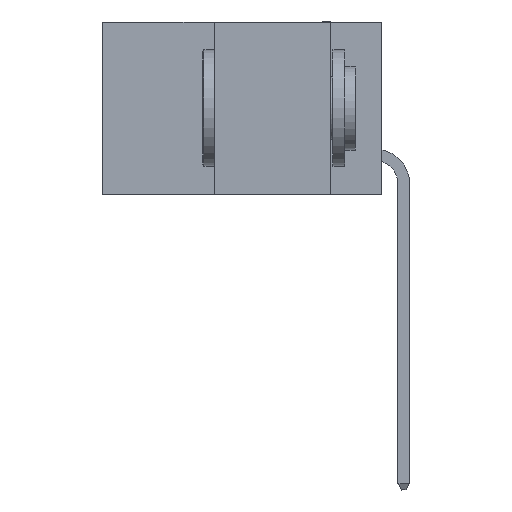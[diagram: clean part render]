
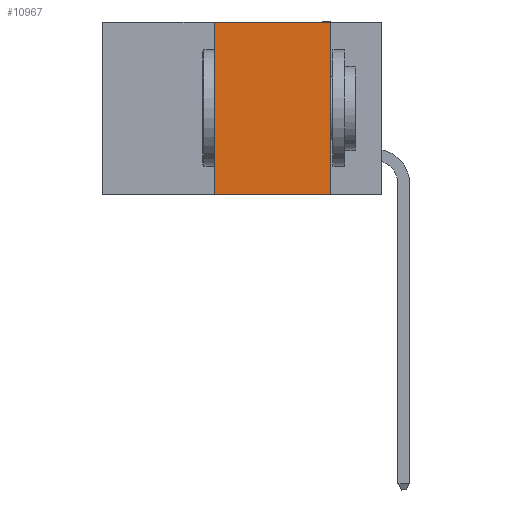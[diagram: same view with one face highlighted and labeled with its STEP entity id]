
A CAD part, left-side view. The second image highlights one B-rep face of the part: STEP entity #10967.
In plain terms, the highlighted planar face has unit normal (-1, 0, 0).
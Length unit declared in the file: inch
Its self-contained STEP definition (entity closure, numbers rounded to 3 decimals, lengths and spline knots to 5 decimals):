
#466 = VECTOR ( 'NONE', #10156, 39.37008 ) ;
#574 = DIRECTION ( 'NONE',  ( 0., 0., 1. ) ) ;
#3462 = CARTESIAN_POINT ( 'NONE',  ( 0., 0.11, -0.37 ) ) ;
#4355 = EDGE_CURVE ( 'NONE', #12598, #27867, #10613, .T. ) ;
#9009 = ORIENTED_EDGE ( 'NONE', *, *, #15326, .F. ) ;
#9457 = CARTESIAN_POINT ( 'NONE',  ( 0., 0.11, 0. ) ) ;
#9523 = DIRECTION ( 'NONE',  ( 1., 0., 0. ) ) ;
#10093 = EDGE_CURVE ( 'NONE', #23717, #25886, #20164, .T. ) ;
#10156 = DIRECTION ( 'NONE',  ( 0., -1., 0. ) ) ;
#10324 = VECTOR ( 'NONE', #28704, 39.37008 ) ;
#10613 = LINE ( 'NONE', #15446, #466 ) ;
#10967 = ADVANCED_FACE ( 'NONE', ( #32724 ), #17359, .F. ) ;
#12266 = VECTOR ( 'NONE', #574, 39.37008 ) ;
#12590 = CARTESIAN_POINT ( 'NONE',  ( 0., 0.6, 0. ) ) ;
#12598 = VERTEX_POINT ( 'NONE', #34914 ) ;
#13986 = CARTESIAN_POINT ( 'NONE',  ( 0., 0.36, 0. ) ) ;
#14071 = CARTESIAN_POINT ( 'NONE',  ( 0., 0.11, 0. ) ) ;
#15326 = EDGE_CURVE ( 'NONE', #25886, #27867, #15802, .T. ) ;
#15446 = CARTESIAN_POINT ( 'NONE',  ( 0., 0.6, -0.37 ) ) ;
#15802 = LINE ( 'NONE', #9457, #10324 ) ;
#17359 = PLANE ( 'NONE',  #34190 ) ;
#19769 = CARTESIAN_POINT ( 'NONE',  ( 0., 0.36, 0. ) ) ;
#20144 = ORIENTED_EDGE ( 'NONE', *, *, #10093, .F. ) ;
#20164 = LINE ( 'NONE', #12590, #30265 ) ;
#23717 = VERTEX_POINT ( 'NONE', #13986 ) ;
#25610 = CARTESIAN_POINT ( 'NONE',  ( 0., 0.6, 0. ) ) ;
#25886 = VERTEX_POINT ( 'NONE', #14071 ) ;
#27046 = EDGE_LOOP ( 'NONE', ( #9009, #20144, #30380, #33128 ) ) ;
#27867 = VERTEX_POINT ( 'NONE', #3462 ) ;
#28590 = EDGE_CURVE ( 'NONE', #12598, #23717, #32447, .T. ) ;
#28704 = DIRECTION ( 'NONE',  ( 0., 0., -1. ) ) ;
#29058 = DIRECTION ( 'NONE',  ( 0., -1., 0. ) ) ;
#30265 = VECTOR ( 'NONE', #29058, 39.37008 ) ;
#30380 = ORIENTED_EDGE ( 'NONE', *, *, #28590, .F. ) ;
#32447 = LINE ( 'NONE', #19769, #12266 ) ;
#32724 = FACE_OUTER_BOUND ( 'NONE', #27046, .T. ) ;
#33128 = ORIENTED_EDGE ( 'NONE', *, *, #4355, .T. ) ;
#33737 = DIRECTION ( 'NONE',  ( 0., 0., -1. ) ) ;
#34190 = AXIS2_PLACEMENT_3D ( 'NONE', #25610, #9523, #33737 ) ;
#34914 = CARTESIAN_POINT ( 'NONE',  ( 0., 0.36, -0.37 ) ) ;
